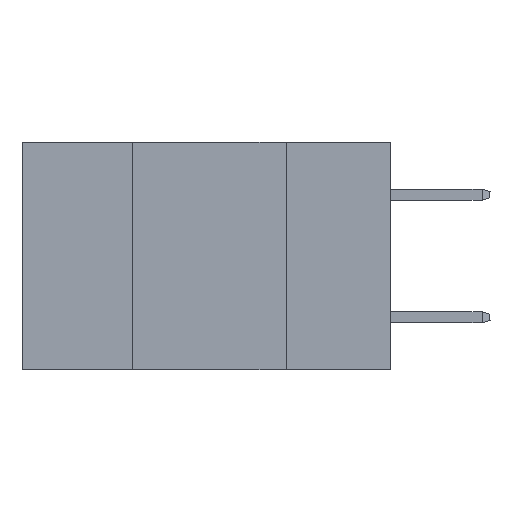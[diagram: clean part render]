
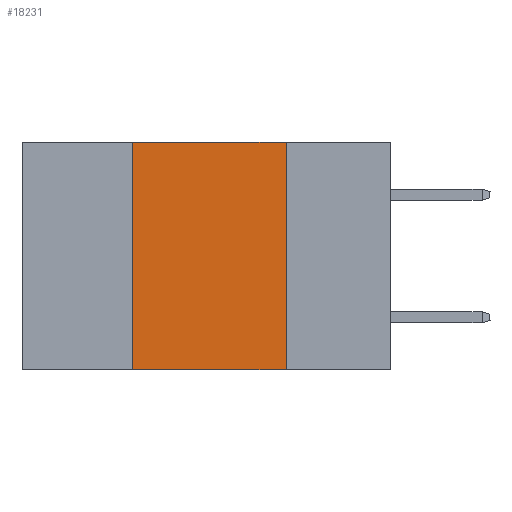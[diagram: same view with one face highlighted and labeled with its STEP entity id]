
A CAD part, left-side view. The second image highlights one B-rep face of the part: STEP entity #18231.
In plain terms, the highlighted planar face has unit normal (-1, 0, 0).
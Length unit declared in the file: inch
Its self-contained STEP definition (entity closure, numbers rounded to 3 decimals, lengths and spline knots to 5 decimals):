
#201 = VERTEX_POINT ( 'NONE', #4800 ) ;
#2342 = ORIENTED_EDGE ( 'NONE', *, *, #2354, .F. ) ;
#2354 = EDGE_CURVE ( 'NONE', #6526, #9978, #15905, .T. ) ;
#2468 = PLANE ( 'NONE',  #3289 ) ;
#2529 = CARTESIAN_POINT ( 'NONE',  ( 0., 0.17, 0. ) ) ;
#2620 = CARTESIAN_POINT ( 'NONE',  ( 0., 0.42, 0. ) ) ;
#3289 = AXIS2_PLACEMENT_3D ( 'NONE', #14766, #4313, #16484 ) ;
#3480 = ORIENTED_EDGE ( 'NONE', *, *, #15763, .F. ) ;
#4313 = DIRECTION ( 'NONE',  ( 1., 0., 0. ) ) ;
#4475 = DIRECTION ( 'NONE',  ( 0., 0., 1. ) ) ;
#4800 = CARTESIAN_POINT ( 'NONE',  ( 0., 0.42, -0.37 ) ) ;
#5112 = VECTOR ( 'NONE', #4475, 39.37008 ) ;
#6074 = LINE ( 'NONE', #19912, #14221 ) ;
#6331 = ORIENTED_EDGE ( 'NONE', *, *, #10772, .F. ) ;
#6526 = VERTEX_POINT ( 'NONE', #8289 ) ;
#6559 = CARTESIAN_POINT ( 'NONE',  ( 0., 0.6, -0.37 ) ) ;
#6843 = EDGE_CURVE ( 'NONE', #201, #7110, #13577, .T. ) ;
#7110 = VERTEX_POINT ( 'NONE', #7980 ) ;
#7980 = CARTESIAN_POINT ( 'NONE',  ( 0., 0.17, -0.37 ) ) ;
#8289 = CARTESIAN_POINT ( 'NONE',  ( 0., 0.42, 0. ) ) ;
#8981 = VECTOR ( 'NONE', #21764, 39.37008 ) ;
#9978 = VERTEX_POINT ( 'NONE', #2529 ) ;
#10772 = EDGE_CURVE ( 'NONE', #201, #6526, #14388, .T. ) ;
#10898 = ORIENTED_EDGE ( 'NONE', *, *, #6843, .T. ) ;
#12407 = EDGE_LOOP ( 'NONE', ( #3480, #2342, #6331, #10898 ) ) ;
#13577 = LINE ( 'NONE', #6559, #8981 ) ;
#14221 = VECTOR ( 'NONE', #21732, 39.37008 ) ;
#14388 = LINE ( 'NONE', #2620, #5112 ) ;
#14766 = CARTESIAN_POINT ( 'NONE',  ( 0., 0.6, 0. ) ) ;
#15214 = CARTESIAN_POINT ( 'NONE',  ( 0., 0.6, 0. ) ) ;
#15598 = DIRECTION ( 'NONE',  ( 0., -1., 0. ) ) ;
#15763 = EDGE_CURVE ( 'NONE', #9978, #7110, #6074, .T. ) ;
#15905 = LINE ( 'NONE', #15214, #16992 ) ;
#16484 = DIRECTION ( 'NONE',  ( 0., 0., -1. ) ) ;
#16992 = VECTOR ( 'NONE', #15598, 39.37008 ) ;
#18231 = ADVANCED_FACE ( 'NONE', ( #22495 ), #2468, .F. ) ;
#19912 = CARTESIAN_POINT ( 'NONE',  ( 0., 0.17, 0. ) ) ;
#21732 = DIRECTION ( 'NONE',  ( 0., 0., -1. ) ) ;
#21764 = DIRECTION ( 'NONE',  ( 0., -1., 0. ) ) ;
#22495 = FACE_OUTER_BOUND ( 'NONE', #12407, .T. ) ;
